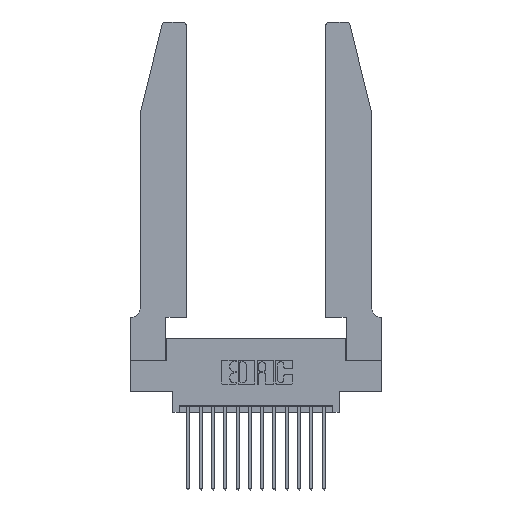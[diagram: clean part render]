
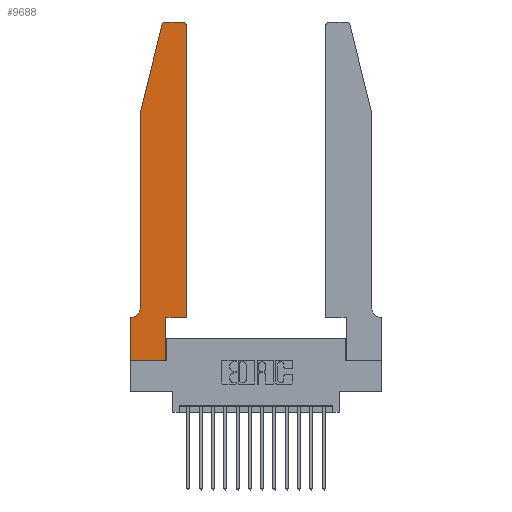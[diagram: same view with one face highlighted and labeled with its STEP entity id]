
A CAD part, top view. The second image highlights one B-rep face of the part: STEP entity #9688.
In plain terms, the highlighted planar face has unit normal (0, 0, 1).
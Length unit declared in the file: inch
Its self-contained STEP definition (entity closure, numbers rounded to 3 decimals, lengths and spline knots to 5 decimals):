
#36 = VERTEX_POINT ( 'NONE', #10679 ) ;
#45 = VECTOR ( 'NONE', #7541, 39.37008 ) ;
#135 = CARTESIAN_POINT ( 'NONE',  ( 0., 0., 0.37 ) ) ;
#166 = VERTEX_POINT ( 'NONE', #16492 ) ;
#232 = CARTESIAN_POINT ( 'NONE',  ( 0.0755, 2., 0.37 ) ) ;
#261 = ORIENTED_EDGE ( 'NONE', *, *, #5230, .T. ) ;
#443 = VERTEX_POINT ( 'NONE', #7410 ) ;
#453 = VERTEX_POINT ( 'NONE', #8042 ) ;
#874 = CIRCLE ( 'NONE', #14424, 0.03 ) ;
#1440 = VERTEX_POINT ( 'NONE', #17596 ) ;
#1625 = PLANE ( 'NONE',  #18188 ) ;
#2020 = LINE ( 'NONE', #232, #16150 ) ;
#2584 = ORIENTED_EDGE ( 'NONE', *, *, #12248, .T. ) ;
#2836 = LINE ( 'NONE', #135, #17388 ) ;
#2866 = EDGE_CURVE ( 'NONE', #9085, #1440, #15931, .T. ) ;
#3082 = DIRECTION ( 'NONE',  ( 0., 0., 1. ) ) ;
#3157 = FACE_OUTER_BOUND ( 'NONE', #10589, .T. ) ;
#3367 = EDGE_CURVE ( 'NONE', #6165, #7190, #874, .T. ) ;
#3381 = VERTEX_POINT ( 'NONE', #5509 ) ;
#3954 = LINE ( 'NONE', #11690, #45 ) ;
#4392 = CIRCLE ( 'NONE', #12993, 0.07 ) ;
#4622 = CARTESIAN_POINT ( 'NONE',  ( 0.2865, 0.35, 0.37 ) ) ;
#4774 = VECTOR ( 'NONE', #11127, 39.37008 ) ;
#5230 = EDGE_CURVE ( 'NONE', #166, #443, #2836, .T. ) ;
#5239 = LINE ( 'NONE', #9721, #4774 ) ;
#5387 = CARTESIAN_POINT ( 'NONE',  ( 0.4205, 2.72, 0.37 ) ) ;
#5415 = DIRECTION ( 'NONE',  ( 1., 0., 0. ) ) ;
#5465 = LINE ( 'NONE', #15889, #6362 ) ;
#5509 = CARTESIAN_POINT ( 'NONE',  ( 0.0755, 2., 0.37 ) ) ;
#6164 = EDGE_CURVE ( 'NONE', #443, #17150, #14485, .T. ) ;
#6165 = VERTEX_POINT ( 'NONE', #10993 ) ;
#6356 = ORIENTED_EDGE ( 'NONE', *, *, #11547, .T. ) ;
#6362 = VECTOR ( 'NONE', #8943, 39.37008 ) ;
#6593 = CARTESIAN_POINT ( 'NONE',  ( 0.2865, 0., 0.37 ) ) ;
#6649 = DIRECTION ( 'NONE',  ( 1., 0., 0. ) ) ;
#6773 = CARTESIAN_POINT ( 'NONE',  ( 0.4505, 0.35, 0.37 ) ) ;
#6819 = DIRECTION ( 'NONE',  ( 1., 0., 0. ) ) ;
#6847 = CARTESIAN_POINT ( 'NONE',  ( 0., 0., 0.37 ) ) ;
#6880 = DIRECTION ( 'NONE',  ( 0., 0., 1. ) ) ;
#7190 = VERTEX_POINT ( 'NONE', #16083 ) ;
#7360 = DIRECTION ( 'NONE',  ( 0., -1., 0. ) ) ;
#7410 = CARTESIAN_POINT ( 'NONE',  ( 0., 0., 0.37 ) ) ;
#7541 = DIRECTION ( 'NONE',  ( -0.239, -0.971, 0. ) ) ;
#7625 = CARTESIAN_POINT ( 'NONE',  ( 0.0055, 0.42, 0.37 ) ) ;
#7717 = ORIENTED_EDGE ( 'NONE', *, *, #11921, .T. ) ;
#7978 = ORIENTED_EDGE ( 'NONE', *, *, #2866, .T. ) ;
#8042 = CARTESIAN_POINT ( 'NONE',  ( 0.4205, 2.75, 0.37 ) ) ;
#8082 = VECTOR ( 'NONE', #6649, 39.37008 ) ;
#8841 = DIRECTION ( 'NONE',  ( 0., -1., 0. ) ) ;
#8943 = DIRECTION ( 'NONE',  ( -1., 0., 0. ) ) ;
#9016 = DIRECTION ( 'NONE',  ( -1., 0., 0. ) ) ;
#9085 = VERTEX_POINT ( 'NONE', #4622 ) ;
#9274 = DIRECTION ( 'NONE',  ( 0., 1., 0. ) ) ;
#9360 = ORIENTED_EDGE ( 'NONE', *, *, #9773, .T. ) ;
#9364 = LINE ( 'NONE', #13068, #16359 ) ;
#9688 = ADVANCED_FACE ( 'NONE', ( #3157 ), #1625, .T. ) ;
#9721 = CARTESIAN_POINT ( 'NONE',  ( 0.4505, 0.35, 0.37 ) ) ;
#9773 = EDGE_CURVE ( 'NONE', #453, #6165, #9364, .T. ) ;
#10589 = EDGE_LOOP ( 'NONE', ( #9360, #11048, #13843, #7717, #17889, #16781, #261, #14861, #6356, #7978, #16503, #2584 ) ) ;
#10679 = CARTESIAN_POINT ( 'NONE',  ( 0.4505, 2.72, 0.37 ) ) ;
#10940 = EDGE_CURVE ( 'NONE', #15342, #166, #5465, .T. ) ;
#10965 = AXIS2_PLACEMENT_3D ( 'NONE', #5387, #15155, #6819 ) ;
#10993 = CARTESIAN_POINT ( 'NONE',  ( 0.284, 2.75, 0.37 ) ) ;
#11048 = ORIENTED_EDGE ( 'NONE', *, *, #3367, .T. ) ;
#11127 = DIRECTION ( 'NONE',  ( 0., 1., 0. ) ) ;
#11219 = EDGE_CURVE ( 'NONE', #1440, #36, #5239, .T. ) ;
#11547 = EDGE_CURVE ( 'NONE', #17150, #9085, #11586, .T. ) ;
#11559 = CARTESIAN_POINT ( 'NONE',  ( 0., 0.35, 0.37 ) ) ;
#11586 = LINE ( 'NONE', #16238, #15270 ) ;
#11690 = CARTESIAN_POINT ( 'NONE',  ( 0.0755, 2., 0.37 ) ) ;
#11921 = EDGE_CURVE ( 'NONE', #3381, #17305, #2020, .T. ) ;
#12248 = EDGE_CURVE ( 'NONE', #36, #453, #14582, .T. ) ;
#12951 = DIRECTION ( 'NONE',  ( 1., 0., 0. ) ) ;
#12993 = AXIS2_PLACEMENT_3D ( 'NONE', #7625, #17401, #9016 ) ;
#13068 = CARTESIAN_POINT ( 'NONE',  ( 0.2605, 2.75, 0.37 ) ) ;
#13843 = ORIENTED_EDGE ( 'NONE', *, *, #18097, .T. ) ;
#14042 = VECTOR ( 'NONE', #5415, 39.37008 ) ;
#14424 = AXIS2_PLACEMENT_3D ( 'NONE', #15213, #6880, #16639 ) ;
#14458 = DIRECTION ( 'NONE',  ( -1., 0., 0. ) ) ;
#14485 = LINE ( 'NONE', #6847, #14042 ) ;
#14582 = CIRCLE ( 'NONE', #10965, 0.03 ) ;
#14861 = ORIENTED_EDGE ( 'NONE', *, *, #6164, .T. ) ;
#15155 = DIRECTION ( 'NONE',  ( 0., 0., 1. ) ) ;
#15213 = CARTESIAN_POINT ( 'NONE',  ( 0.284, 2.72, 0.37 ) ) ;
#15236 = CARTESIAN_POINT ( 'NONE',  ( 0.0755, 0.42, 0.37 ) ) ;
#15270 = VECTOR ( 'NONE', #9274, 39.37008 ) ;
#15342 = VERTEX_POINT ( 'NONE', #16207 ) ;
#15889 = CARTESIAN_POINT ( 'NONE',  ( 0.0755, 0.35, 0.37 ) ) ;
#15931 = LINE ( 'NONE', #6773, #8082 ) ;
#16083 = CARTESIAN_POINT ( 'NONE',  ( 0.25487, 2.72718, 0.37 ) ) ;
#16150 = VECTOR ( 'NONE', #8841, 39.37008 ) ;
#16207 = CARTESIAN_POINT ( 'NONE',  ( 0.0055, 0.35, 0.37 ) ) ;
#16238 = CARTESIAN_POINT ( 'NONE',  ( 0.2865, 0.35, 0.37 ) ) ;
#16359 = VECTOR ( 'NONE', #14458, 39.37008 ) ;
#16451 = EDGE_CURVE ( 'NONE', #17305, #15342, #4392, .T. ) ;
#16492 = CARTESIAN_POINT ( 'NONE',  ( 0., 0.35, 0.37 ) ) ;
#16503 = ORIENTED_EDGE ( 'NONE', *, *, #11219, .T. ) ;
#16639 = DIRECTION ( 'NONE',  ( 1., 0., 0. ) ) ;
#16781 = ORIENTED_EDGE ( 'NONE', *, *, #10940, .T. ) ;
#17150 = VERTEX_POINT ( 'NONE', #6593 ) ;
#17305 = VERTEX_POINT ( 'NONE', #15236 ) ;
#17388 = VECTOR ( 'NONE', #7360, 39.37008 ) ;
#17401 = DIRECTION ( 'NONE',  ( 0., 0., -1. ) ) ;
#17596 = CARTESIAN_POINT ( 'NONE',  ( 0.4505, 0.35, 0.37 ) ) ;
#17889 = ORIENTED_EDGE ( 'NONE', *, *, #16451, .T. ) ;
#18097 = EDGE_CURVE ( 'NONE', #7190, #3381, #3954, .T. ) ;
#18188 = AXIS2_PLACEMENT_3D ( 'NONE', #11559, #3082, #12951 ) ;
